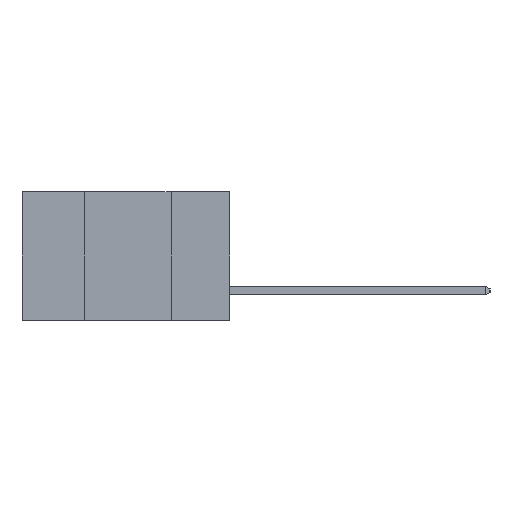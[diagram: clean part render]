
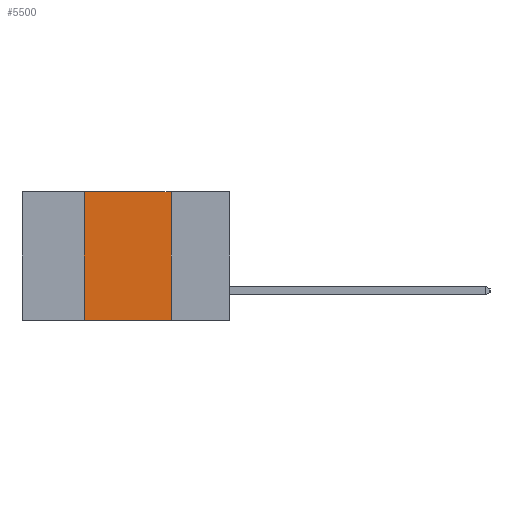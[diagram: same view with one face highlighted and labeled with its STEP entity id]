
A CAD part, left-side view. The second image highlights one B-rep face of the part: STEP entity #5500.
In plain terms, the highlighted planar face has unit normal (-1, 0, 0).
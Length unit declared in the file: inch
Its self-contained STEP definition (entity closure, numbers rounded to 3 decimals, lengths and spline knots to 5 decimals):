
#48 = LINE ( 'NONE', #7058, #14962 ) ;
#1105 = VERTEX_POINT ( 'NONE', #16220 ) ;
#1208 = DIRECTION ( 'NONE',  ( 0., 0., 1. ) ) ;
#3026 = EDGE_LOOP ( 'NONE', ( #6560, #3387, #5912, #10996 ) ) ;
#3103 = DIRECTION ( 'NONE',  ( 0., -1., 0. ) ) ;
#3307 = VECTOR ( 'NONE', #10168, 39.37008 ) ;
#3387 = ORIENTED_EDGE ( 'NONE', *, *, #12146, .F. ) ;
#4095 = CARTESIAN_POINT ( 'NONE',  ( 0., 0.6, 0. ) ) ;
#4282 = VECTOR ( 'NONE', #3103, 39.37008 ) ;
#4762 = FACE_OUTER_BOUND ( 'NONE', #3026, .T. ) ;
#5500 = ADVANCED_FACE ( 'NONE', ( #4762 ), #13369, .F. ) ;
#5556 = DIRECTION ( 'NONE',  ( 0., 0., -1. ) ) ;
#5571 = DIRECTION ( 'NONE',  ( 0., -1., 0. ) ) ;
#5912 = ORIENTED_EDGE ( 'NONE', *, *, #15457, .F. ) ;
#6560 = ORIENTED_EDGE ( 'NONE', *, *, #17574, .F. ) ;
#7058 = CARTESIAN_POINT ( 'NONE',  ( 0., 0.42, 0. ) ) ;
#8732 = CARTESIAN_POINT ( 'NONE',  ( 0., 0.17, 0. ) ) ;
#9648 = AXIS2_PLACEMENT_3D ( 'NONE', #16531, #12863, #5556 ) ;
#10168 = DIRECTION ( 'NONE',  ( 0., 0., -1. ) ) ;
#10524 = VERTEX_POINT ( 'NONE', #16153 ) ;
#10922 = CARTESIAN_POINT ( 'NONE',  ( 0., 0.42, 0. ) ) ;
#10996 = ORIENTED_EDGE ( 'NONE', *, *, #18143, .T. ) ;
#11292 = VERTEX_POINT ( 'NONE', #10922 ) ;
#11348 = LINE ( 'NONE', #8732, #3307 ) ;
#12146 = EDGE_CURVE ( 'NONE', #11292, #1105, #16318, .T. ) ;
#12659 = VECTOR ( 'NONE', #5571, 39.37008 ) ;
#12863 = DIRECTION ( 'NONE',  ( 1., 0., 0. ) ) ;
#13369 = PLANE ( 'NONE',  #9648 ) ;
#14048 = VERTEX_POINT ( 'NONE', #15217 ) ;
#14454 = CARTESIAN_POINT ( 'NONE',  ( 0., 0.6, -0.37 ) ) ;
#14962 = VECTOR ( 'NONE', #1208, 39.37008 ) ;
#15173 = LINE ( 'NONE', #14454, #4282 ) ;
#15217 = CARTESIAN_POINT ( 'NONE',  ( 0., 0.17, -0.37 ) ) ;
#15457 = EDGE_CURVE ( 'NONE', #10524, #11292, #48, .T. ) ;
#16153 = CARTESIAN_POINT ( 'NONE',  ( 0., 0.42, -0.37 ) ) ;
#16220 = CARTESIAN_POINT ( 'NONE',  ( 0., 0.17, 0. ) ) ;
#16318 = LINE ( 'NONE', #4095, #12659 ) ;
#16531 = CARTESIAN_POINT ( 'NONE',  ( 0., 0.6, 0. ) ) ;
#17574 = EDGE_CURVE ( 'NONE', #1105, #14048, #11348, .T. ) ;
#18143 = EDGE_CURVE ( 'NONE', #10524, #14048, #15173, .T. ) ;
